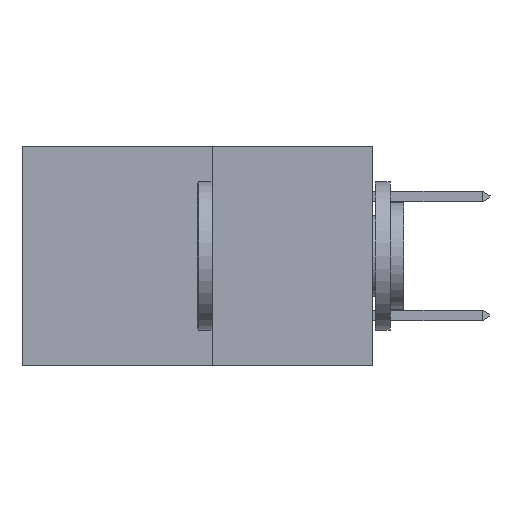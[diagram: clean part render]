
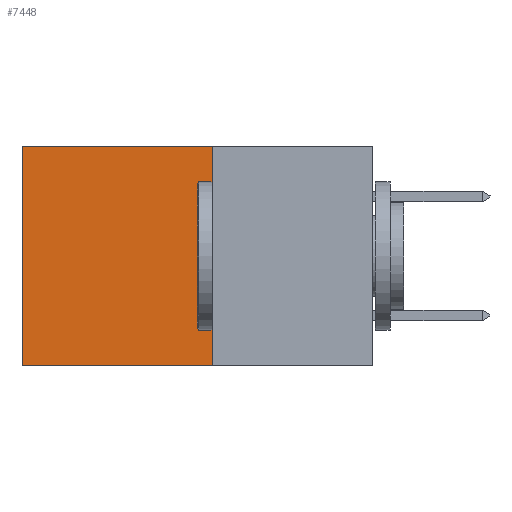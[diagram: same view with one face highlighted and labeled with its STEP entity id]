
A CAD part, left-side view. The second image highlights one B-rep face of the part: STEP entity #7448.
In plain terms, the highlighted planar face has unit normal (-1, 0, 0).
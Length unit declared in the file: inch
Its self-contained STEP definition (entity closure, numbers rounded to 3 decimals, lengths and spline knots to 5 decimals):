
#530 = DIRECTION ( 'NONE',  ( 0., 1., 0. ) ) ;
#1631 = LINE ( 'NONE', #8328, #12110 ) ;
#1760 = EDGE_CURVE ( 'NONE', #3385, #3325, #1631, .T. ) ;
#2083 = EDGE_CURVE ( 'NONE', #15380, #3325, #16682, .T. ) ;
#2394 = CARTESIAN_POINT ( 'NONE',  ( 0.277, 0.27, -0.37 ) ) ;
#2466 = LINE ( 'NONE', #5822, #16286 ) ;
#2548 = FACE_OUTER_BOUND ( 'NONE', #5049, .T. ) ;
#3190 = CARTESIAN_POINT ( 'NONE',  ( 0.277, 0.27, 0. ) ) ;
#3229 = DIRECTION ( 'NONE',  ( 0., 0., -1. ) ) ;
#3325 = VERTEX_POINT ( 'NONE', #13519 ) ;
#3385 = VERTEX_POINT ( 'NONE', #5350 ) ;
#3697 = VECTOR ( 'NONE', #7701, 39.37008 ) ;
#4554 = DIRECTION ( 'NONE',  ( 0., 1., 0. ) ) ;
#5022 = DIRECTION ( 'NONE',  ( 1., 0., 0. ) ) ;
#5049 = EDGE_LOOP ( 'NONE', ( #11739, #11332, #14393, #10899 ) ) ;
#5051 = CARTESIAN_POINT ( 'NONE',  ( 0.277, 0.27, 0. ) ) ;
#5350 = CARTESIAN_POINT ( 'NONE',  ( 0.277, 0.27, -0.37 ) ) ;
#5822 = CARTESIAN_POINT ( 'NONE',  ( 0.277, 0.27, -0.37 ) ) ;
#7448 = ADVANCED_FACE ( 'NONE', ( #2548 ), #16652, .F. ) ;
#7701 = DIRECTION ( 'NONE',  ( 0., 0., -1. ) ) ;
#8328 = CARTESIAN_POINT ( 'NONE',  ( 0.277, 0.27, -0.37 ) ) ;
#10591 = EDGE_CURVE ( 'NONE', #11586, #3385, #2466, .T. ) ;
#10899 = ORIENTED_EDGE ( 'NONE', *, *, #11997, .T. ) ;
#11332 = ORIENTED_EDGE ( 'NONE', *, *, #1760, .F. ) ;
#11586 = VERTEX_POINT ( 'NONE', #5051 ) ;
#11739 = ORIENTED_EDGE ( 'NONE', *, *, #2083, .T. ) ;
#11997 = EDGE_CURVE ( 'NONE', #11586, #15380, #15841, .T. ) ;
#12110 = VECTOR ( 'NONE', #530, 39.37008 ) ;
#12452 = VECTOR ( 'NONE', #4554, 39.37008 ) ;
#13058 = CARTESIAN_POINT ( 'NONE',  ( 0.277, 0.59, 0. ) ) ;
#13519 = CARTESIAN_POINT ( 'NONE',  ( 0.277, 0.59, -0.37 ) ) ;
#13824 = AXIS2_PLACEMENT_3D ( 'NONE', #2394, #5022, #14216 ) ;
#13874 = CARTESIAN_POINT ( 'NONE',  ( 0.277, 0.59, -0.37 ) ) ;
#14216 = DIRECTION ( 'NONE',  ( 0., 0., -1. ) ) ;
#14393 = ORIENTED_EDGE ( 'NONE', *, *, #10591, .F. ) ;
#15380 = VERTEX_POINT ( 'NONE', #13058 ) ;
#15841 = LINE ( 'NONE', #3190, #12452 ) ;
#16286 = VECTOR ( 'NONE', #3229, 39.37008 ) ;
#16652 = PLANE ( 'NONE',  #13824 ) ;
#16682 = LINE ( 'NONE', #13874, #3697 ) ;
